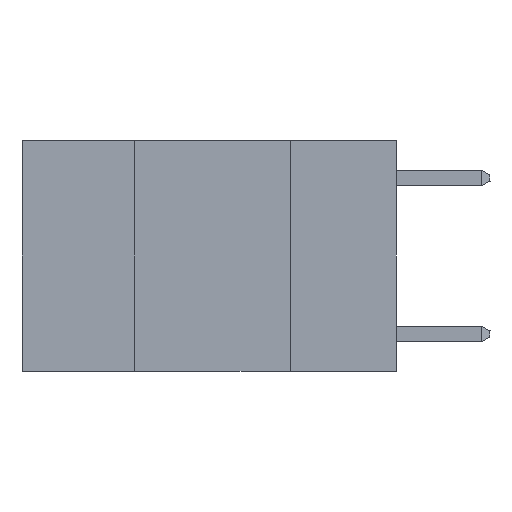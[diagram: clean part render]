
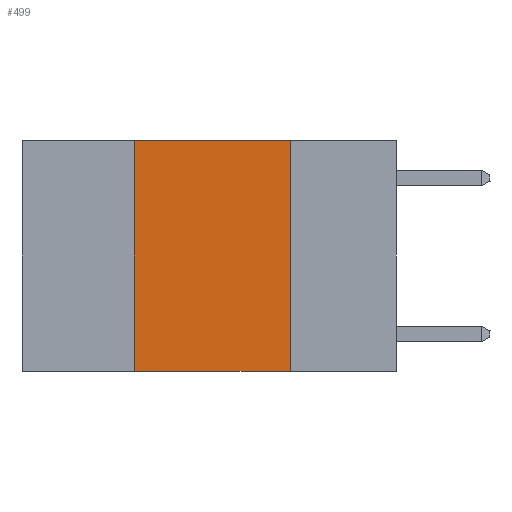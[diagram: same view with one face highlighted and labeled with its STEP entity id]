
A CAD part, left-side view. The second image highlights one B-rep face of the part: STEP entity #499.
In plain terms, the highlighted planar face has unit normal (-1, 0, 0).
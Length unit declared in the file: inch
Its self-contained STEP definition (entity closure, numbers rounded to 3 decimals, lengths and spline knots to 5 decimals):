
#394 = VERTEX_POINT ( 'NONE', #10877 ) ;
#499 = ADVANCED_FACE ( 'NONE', ( #4293 ), #3413, .F. ) ;
#663 = EDGE_CURVE ( 'NONE', #394, #10161, #3124, .T. ) ;
#846 = ORIENTED_EDGE ( 'NONE', *, *, #11359, .T. ) ;
#993 = ORIENTED_EDGE ( 'NONE', *, *, #663, .F. ) ;
#1453 = CARTESIAN_POINT ( 'NONE',  ( 0., 0.17, 0. ) ) ;
#1782 = VECTOR ( 'NONE', #5121, 39.37008 ) ;
#1882 = EDGE_CURVE ( 'NONE', #7890, #394, #8708, .T. ) ;
#2174 = AXIS2_PLACEMENT_3D ( 'NONE', #3952, #4961, #6415 ) ;
#2870 = VECTOR ( 'NONE', #12251, 39.37008 ) ;
#3051 = ORIENTED_EDGE ( 'NONE', *, *, #10433, .F. ) ;
#3124 = LINE ( 'NONE', #1453, #2870 ) ;
#3337 = VERTEX_POINT ( 'NONE', #12149 ) ;
#3413 = PLANE ( 'NONE',  #2174 ) ;
#3952 = CARTESIAN_POINT ( 'NONE',  ( 0., 0.6, 0. ) ) ;
#4081 = CARTESIAN_POINT ( 'NONE',  ( 0., 0.42, 0. ) ) ;
#4293 = FACE_OUTER_BOUND ( 'NONE', #12277, .T. ) ;
#4455 = CARTESIAN_POINT ( 'NONE',  ( 0., 0.6, -0.37 ) ) ;
#4961 = DIRECTION ( 'NONE',  ( 1., 0., 0. ) ) ;
#5121 = DIRECTION ( 'NONE',  ( 0., 0., 1. ) ) ;
#6415 = DIRECTION ( 'NONE',  ( 0., 0., -1. ) ) ;
#6572 = DIRECTION ( 'NONE',  ( 0., -1., 0. ) ) ;
#6574 = ORIENTED_EDGE ( 'NONE', *, *, #1882, .F. ) ;
#6607 = CARTESIAN_POINT ( 'NONE',  ( 0., 0.17, -0.37 ) ) ;
#6937 = LINE ( 'NONE', #4455, #11791 ) ;
#7636 = CARTESIAN_POINT ( 'NONE',  ( 0., 0.6, 0. ) ) ;
#7890 = VERTEX_POINT ( 'NONE', #11327 ) ;
#8708 = LINE ( 'NONE', #7636, #10736 ) ;
#9241 = DIRECTION ( 'NONE',  ( 0., -1., 0. ) ) ;
#10161 = VERTEX_POINT ( 'NONE', #6607 ) ;
#10400 = LINE ( 'NONE', #4081, #1782 ) ;
#10433 = EDGE_CURVE ( 'NONE', #3337, #7890, #10400, .T. ) ;
#10736 = VECTOR ( 'NONE', #6572, 39.37008 ) ;
#10877 = CARTESIAN_POINT ( 'NONE',  ( 0., 0.17, 0. ) ) ;
#11327 = CARTESIAN_POINT ( 'NONE',  ( 0., 0.42, 0. ) ) ;
#11359 = EDGE_CURVE ( 'NONE', #3337, #10161, #6937, .T. ) ;
#11791 = VECTOR ( 'NONE', #9241, 39.37008 ) ;
#12149 = CARTESIAN_POINT ( 'NONE',  ( 0., 0.42, -0.37 ) ) ;
#12251 = DIRECTION ( 'NONE',  ( 0., 0., -1. ) ) ;
#12277 = EDGE_LOOP ( 'NONE', ( #993, #6574, #3051, #846 ) ) ;
